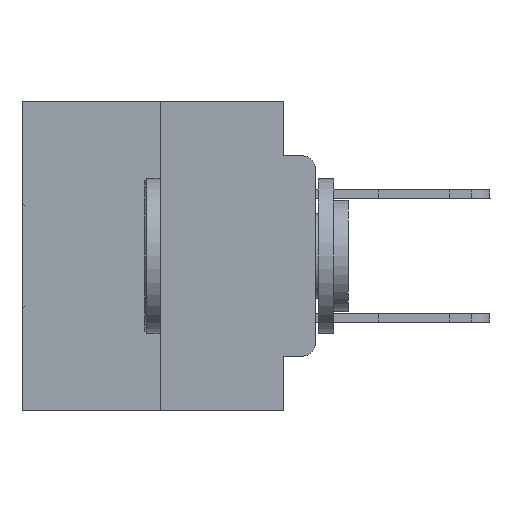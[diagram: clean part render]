
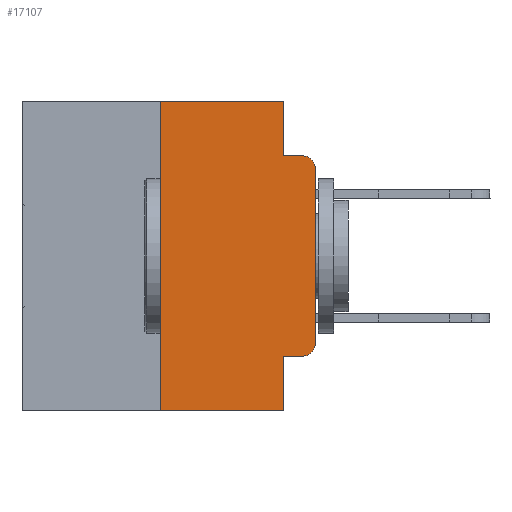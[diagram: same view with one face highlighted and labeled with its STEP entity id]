
A CAD part, left-side view. The second image highlights one B-rep face of the part: STEP entity #17107.
In plain terms, the highlighted planar face has unit normal (-1, 0, 0).
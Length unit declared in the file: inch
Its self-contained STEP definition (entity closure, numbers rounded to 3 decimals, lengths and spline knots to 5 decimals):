
#125 = VECTOR ( 'NONE', #27692, 39.37008 ) ;
#335 = DIRECTION ( 'NONE',  ( 0., -1., 0. ) ) ;
#3075 = EDGE_CURVE ( 'NONE', #9514, #9971, #6650, .T. ) ;
#3311 = EDGE_CURVE ( 'NONE', #7917, #16025, #6327, .T. ) ;
#3593 = DIRECTION ( 'NONE',  ( 0., 0., -1. ) ) ;
#3761 = LINE ( 'NONE', #16806, #32118 ) ;
#3843 = AXIS2_PLACEMENT_3D ( 'NONE', #29184, #6844, #16764 ) ;
#3971 = CARTESIAN_POINT ( 'NONE',  ( 0., 0.051, -0.5 ) ) ;
#4687 = VERTEX_POINT ( 'NONE', #19105 ) ;
#6327 = LINE ( 'NONE', #13490, #31151 ) ;
#6650 = CIRCLE ( 'NONE', #17024, 0.02 ) ;
#6844 = DIRECTION ( 'NONE',  ( 1., 0., 0. ) ) ;
#7790 = AXIS2_PLACEMENT_3D ( 'NONE', #21369, #25963, #3593 ) ;
#7805 = CARTESIAN_POINT ( 'NONE',  ( 0., 0., 0. ) ) ;
#7917 = VERTEX_POINT ( 'NONE', #26699 ) ;
#9038 = EDGE_CURVE ( 'NONE', #7917, #29429, #23590, .T. ) ;
#9302 = FACE_OUTER_BOUND ( 'NONE', #26030, .T. ) ;
#9514 = VERTEX_POINT ( 'NONE', #13945 ) ;
#9717 = VERTEX_POINT ( 'NONE', #12771 ) ;
#9971 = VERTEX_POINT ( 'NONE', #19123 ) ;
#9973 = DIRECTION ( 'NONE',  ( 0., -1., 0. ) ) ;
#10515 = VECTOR ( 'NONE', #26232, 39.37008 ) ;
#11381 = ORIENTED_EDGE ( 'NONE', *, *, #3311, .F. ) ;
#11740 = DIRECTION ( 'NONE',  ( 0., -1., 0. ) ) ;
#11808 = ORIENTED_EDGE ( 'NONE', *, *, #9038, .T. ) ;
#12137 = EDGE_CURVE ( 'NONE', #4687, #21788, #26004, .T. ) ;
#12156 = VECTOR ( 'NONE', #11740, 39.37008 ) ;
#12222 = LINE ( 'NONE', #32128, #12156 ) ;
#12344 = LINE ( 'NONE', #25056, #30228 ) ;
#12586 = EDGE_CURVE ( 'NONE', #9717, #28713, #18178, .T. ) ;
#12771 = CARTESIAN_POINT ( 'NONE',  ( 0., 0.02, -0.4115 ) ) ;
#12821 = DIRECTION ( 'NONE',  ( 0., 0., -1. ) ) ;
#13151 = DIRECTION ( 'NONE',  ( 0., 0., 1. ) ) ;
#13219 = EDGE_CURVE ( 'NONE', #26192, #29429, #12344, .T. ) ;
#13490 = CARTESIAN_POINT ( 'NONE',  ( 0., 0.25, 0. ) ) ;
#13656 = CARTESIAN_POINT ( 'NONE',  ( 0., 0.473, -0.5 ) ) ;
#13708 = CARTESIAN_POINT ( 'NONE',  ( 0., 0.02, -0.1085 ) ) ;
#13945 = CARTESIAN_POINT ( 'NONE',  ( 0., 0., -0.1085 ) ) ;
#14118 = ORIENTED_EDGE ( 'NONE', *, *, #12586, .T. ) ;
#16025 = VERTEX_POINT ( 'NONE', #16844 ) ;
#16764 = DIRECTION ( 'NONE',  ( 0., 0., -1. ) ) ;
#16806 = CARTESIAN_POINT ( 'NONE',  ( 0., 0.051, -0.0885 ) ) ;
#16844 = CARTESIAN_POINT ( 'NONE',  ( 0., 0.25, 0. ) ) ;
#17024 = AXIS2_PLACEMENT_3D ( 'NONE', #13708, #20553, #25807 ) ;
#17107 = ADVANCED_FACE ( 'NONE', ( #9302 ), #19223, .F. ) ;
#17498 = VECTOR ( 'NONE', #18648, 39.37008 ) ;
#17821 = VECTOR ( 'NONE', #335, 39.37008 ) ;
#18163 = CARTESIAN_POINT ( 'NONE',  ( 0., 0.051, -0.4115 ) ) ;
#18178 = CIRCLE ( 'NONE', #7790, 0.02 ) ;
#18334 = EDGE_CURVE ( 'NONE', #26192, #9717, #12222, .T. ) ;
#18559 = EDGE_CURVE ( 'NONE', #28713, #9514, #28621, .T. ) ;
#18648 = DIRECTION ( 'NONE',  ( 0., 0., -1. ) ) ;
#19105 = CARTESIAN_POINT ( 'NONE',  ( 0., 0.051, 0. ) ) ;
#19123 = CARTESIAN_POINT ( 'NONE',  ( 0., 0.02, -0.0885 ) ) ;
#19223 = PLANE ( 'NONE',  #3843 ) ;
#19925 = CARTESIAN_POINT ( 'NONE',  ( 0., 0.473, 0. ) ) ;
#20553 = DIRECTION ( 'NONE',  ( -1., 0., 0. ) ) ;
#21060 = ORIENTED_EDGE ( 'NONE', *, *, #31395, .F. ) ;
#21369 = CARTESIAN_POINT ( 'NONE',  ( 0., 0.02, -0.3915 ) ) ;
#21788 = VERTEX_POINT ( 'NONE', #26829 ) ;
#22856 = LINE ( 'NONE', #19925, #17821 ) ;
#23356 = ORIENTED_EDGE ( 'NONE', *, *, #13219, .F. ) ;
#23590 = LINE ( 'NONE', #13656, #10515 ) ;
#25056 = CARTESIAN_POINT ( 'NONE',  ( 0., 0.051, 0. ) ) ;
#25807 = DIRECTION ( 'NONE',  ( 0., 0., -1. ) ) ;
#25963 = DIRECTION ( 'NONE',  ( -1., 0., 0. ) ) ;
#26004 = LINE ( 'NONE', #30910, #17498 ) ;
#26030 = EDGE_LOOP ( 'NONE', ( #27137, #26219, #21060, #31104, #31832, #11381, #11808, #23356, #26859, #14118 ) ) ;
#26192 = VERTEX_POINT ( 'NONE', #18163 ) ;
#26219 = ORIENTED_EDGE ( 'NONE', *, *, #3075, .T. ) ;
#26232 = DIRECTION ( 'NONE',  ( 0., -1., 0. ) ) ;
#26596 = EDGE_CURVE ( 'NONE', #16025, #4687, #22856, .T. ) ;
#26699 = CARTESIAN_POINT ( 'NONE',  ( 0., 0.25, -0.5 ) ) ;
#26829 = CARTESIAN_POINT ( 'NONE',  ( 0., 0.051, -0.0885 ) ) ;
#26859 = ORIENTED_EDGE ( 'NONE', *, *, #18334, .T. ) ;
#27137 = ORIENTED_EDGE ( 'NONE', *, *, #18559, .T. ) ;
#27692 = DIRECTION ( 'NONE',  ( 0., 0., 1. ) ) ;
#28621 = LINE ( 'NONE', #7805, #125 ) ;
#28713 = VERTEX_POINT ( 'NONE', #31659 ) ;
#29184 = CARTESIAN_POINT ( 'NONE',  ( 0., 0.473, 0. ) ) ;
#29429 = VERTEX_POINT ( 'NONE', #3971 ) ;
#30228 = VECTOR ( 'NONE', #12821, 39.37008 ) ;
#30910 = CARTESIAN_POINT ( 'NONE',  ( 0., 0.051, 0. ) ) ;
#31104 = ORIENTED_EDGE ( 'NONE', *, *, #12137, .F. ) ;
#31151 = VECTOR ( 'NONE', #13151, 39.37008 ) ;
#31395 = EDGE_CURVE ( 'NONE', #21788, #9971, #3761, .T. ) ;
#31659 = CARTESIAN_POINT ( 'NONE',  ( 0., 0., -0.3915 ) ) ;
#31832 = ORIENTED_EDGE ( 'NONE', *, *, #26596, .F. ) ;
#32118 = VECTOR ( 'NONE', #9973, 39.37008 ) ;
#32128 = CARTESIAN_POINT ( 'NONE',  ( 0., 0.051, -0.4115 ) ) ;
